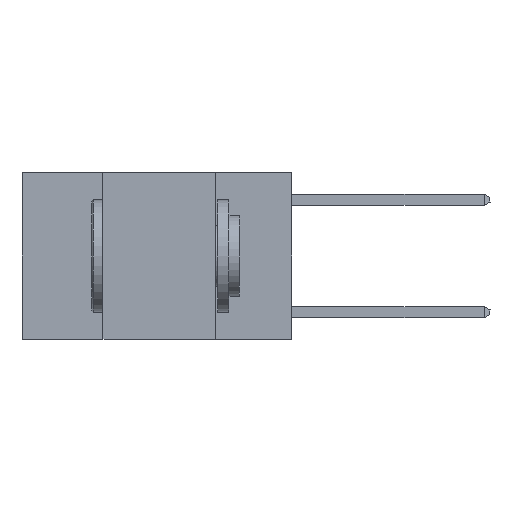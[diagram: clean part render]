
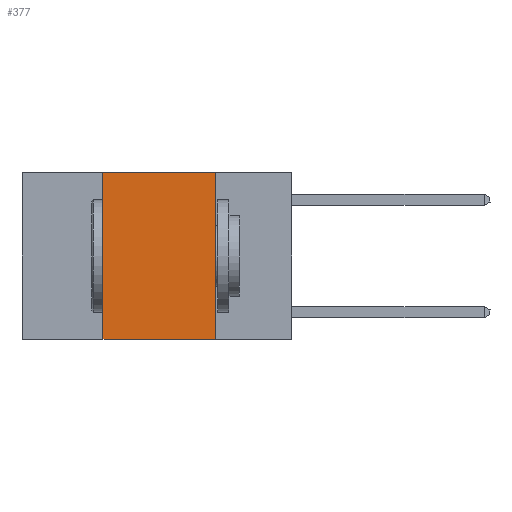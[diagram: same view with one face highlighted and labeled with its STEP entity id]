
A CAD part, left-side view. The second image highlights one B-rep face of the part: STEP entity #377.
In plain terms, the highlighted planar face has unit normal (-1, 0, 0).
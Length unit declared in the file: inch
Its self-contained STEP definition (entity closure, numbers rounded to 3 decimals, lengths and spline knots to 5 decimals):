
#116 = PLANE ( 'NONE',  #1522 ) ;
#377 = ADVANCED_FACE ( 'NONE', ( #6698 ), #116, .F. ) ;
#866 = CARTESIAN_POINT ( 'NONE',  ( 0., 0.17, 0. ) ) ;
#1010 = EDGE_CURVE ( 'NONE', #9215, #1102, #3429, .T. ) ;
#1102 = VERTEX_POINT ( 'NONE', #8165 ) ;
#1289 = CARTESIAN_POINT ( 'NONE',  ( 0., 0.42, 0. ) ) ;
#1522 = AXIS2_PLACEMENT_3D ( 'NONE', #7869, #3805, #3774 ) ;
#1695 = VECTOR ( 'NONE', #2257, 39.37008 ) ;
#1792 = VECTOR ( 'NONE', #3744, 39.37008 ) ;
#2257 = DIRECTION ( 'NONE',  ( 0., -1., 0. ) ) ;
#2548 = ORIENTED_EDGE ( 'NONE', *, *, #8549, .T. ) ;
#3036 = CARTESIAN_POINT ( 'NONE',  ( 0., 0.6, -0.37 ) ) ;
#3429 = LINE ( 'NONE', #5703, #1695 ) ;
#3463 = LINE ( 'NONE', #8276, #9042 ) ;
#3744 = DIRECTION ( 'NONE',  ( 0., -1., 0. ) ) ;
#3774 = DIRECTION ( 'NONE',  ( 0., 0., -1. ) ) ;
#3805 = DIRECTION ( 'NONE',  ( 1., 0., 0. ) ) ;
#3935 = VECTOR ( 'NONE', #6046, 39.37008 ) ;
#4464 = ORIENTED_EDGE ( 'NONE', *, *, #5622, .F. ) ;
#4488 = CARTESIAN_POINT ( 'NONE',  ( 0., 0.42, -0.37 ) ) ;
#4616 = DIRECTION ( 'NONE',  ( 0., 0., 1. ) ) ;
#5124 = ORIENTED_EDGE ( 'NONE', *, *, #1010, .F. ) ;
#5181 = ORIENTED_EDGE ( 'NONE', *, *, #9522, .F. ) ;
#5399 = VERTEX_POINT ( 'NONE', #4488 ) ;
#5622 = EDGE_CURVE ( 'NONE', #5399, #9215, #3463, .T. ) ;
#5681 = LINE ( 'NONE', #3036, #1792 ) ;
#5703 = CARTESIAN_POINT ( 'NONE',  ( 0., 0.6, 0. ) ) ;
#5805 = EDGE_LOOP ( 'NONE', ( #5181, #5124, #4464, #2548 ) ) ;
#5890 = LINE ( 'NONE', #866, #3935 ) ;
#6046 = DIRECTION ( 'NONE',  ( 0., 0., -1. ) ) ;
#6698 = FACE_OUTER_BOUND ( 'NONE', #5805, .T. ) ;
#7869 = CARTESIAN_POINT ( 'NONE',  ( 0., 0.6, 0. ) ) ;
#8165 = CARTESIAN_POINT ( 'NONE',  ( 0., 0.17, 0. ) ) ;
#8276 = CARTESIAN_POINT ( 'NONE',  ( 0., 0.42, 0. ) ) ;
#8549 = EDGE_CURVE ( 'NONE', #5399, #8561, #5681, .T. ) ;
#8561 = VERTEX_POINT ( 'NONE', #9521 ) ;
#9042 = VECTOR ( 'NONE', #4616, 39.37008 ) ;
#9215 = VERTEX_POINT ( 'NONE', #1289 ) ;
#9521 = CARTESIAN_POINT ( 'NONE',  ( 0., 0.17, -0.37 ) ) ;
#9522 = EDGE_CURVE ( 'NONE', #1102, #8561, #5890, .T. ) ;
